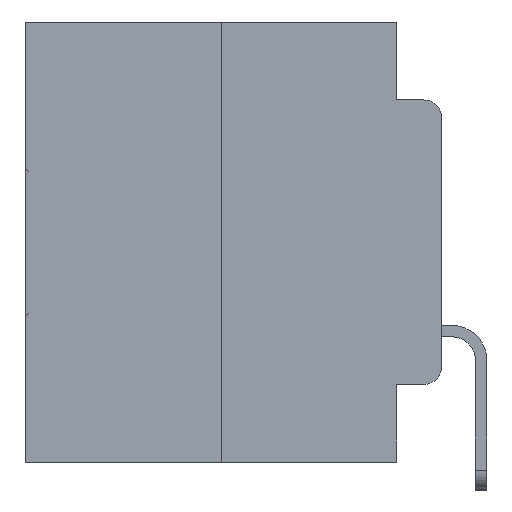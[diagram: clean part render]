
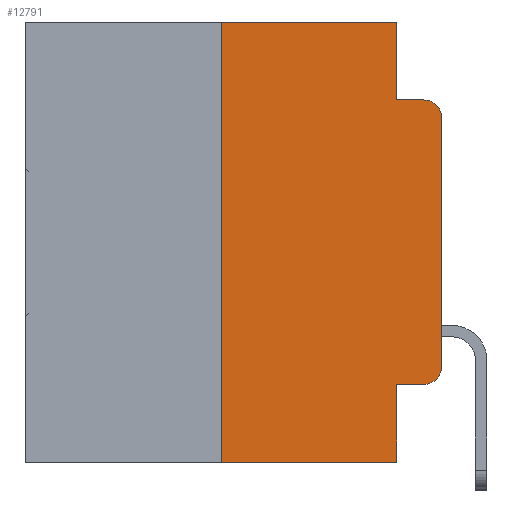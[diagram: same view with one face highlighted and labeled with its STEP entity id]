
A CAD part, left-side view. The second image highlights one B-rep face of the part: STEP entity #12791.
In plain terms, the highlighted planar face has unit normal (-1, 0, 0).
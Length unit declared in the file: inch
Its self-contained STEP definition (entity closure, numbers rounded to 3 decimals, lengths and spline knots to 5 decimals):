
#526 = DIRECTION ( 'NONE',  ( 0., -1., 0. ) ) ;
#586 = DIRECTION ( 'NONE',  ( 0., 0., -1. ) ) ;
#830 = CARTESIAN_POINT ( 'NONE',  ( 0., 0.02, -0.4115 ) ) ;
#928 = EDGE_CURVE ( 'NONE', #4862, #18999, #29889, .T. ) ;
#1311 = DIRECTION ( 'NONE',  ( -1., 0., 0. ) ) ;
#1475 = VECTOR ( 'NONE', #29833, 39.37008 ) ;
#1759 = CARTESIAN_POINT ( 'NONE',  ( 0., 0.473, -0.5 ) ) ;
#2125 = VERTEX_POINT ( 'NONE', #4407 ) ;
#2198 = FACE_OUTER_BOUND ( 'NONE', #23695, .T. ) ;
#2597 = LINE ( 'NONE', #1759, #7524 ) ;
#2882 = EDGE_CURVE ( 'NONE', #18999, #2125, #15155, .T. ) ;
#4063 = CARTESIAN_POINT ( 'NONE',  ( 0., 0.02, -0.0885 ) ) ;
#4392 = CARTESIAN_POINT ( 'NONE',  ( 0., 0., -0.3915 ) ) ;
#4407 = CARTESIAN_POINT ( 'NONE',  ( 0., 0., -0.1085 ) ) ;
#4862 = VERTEX_POINT ( 'NONE', #830 ) ;
#7303 = ORIENTED_EDGE ( 'NONE', *, *, #928, .T. ) ;
#7524 = VECTOR ( 'NONE', #16110, 39.37008 ) ;
#9722 = VECTOR ( 'NONE', #9874, 39.37008 ) ;
#9874 = DIRECTION ( 'NONE',  ( 0., 0., -1. ) ) ;
#9899 = DIRECTION ( 'NONE',  ( -1., 0., 0. ) ) ;
#10083 = VERTEX_POINT ( 'NONE', #19619 ) ;
#10897 = AXIS2_PLACEMENT_3D ( 'NONE', #15688, #1311, #18074 ) ;
#10962 = ORIENTED_EDGE ( 'NONE', *, *, #14187, .F. ) ;
#11020 = ORIENTED_EDGE ( 'NONE', *, *, #17382, .F. ) ;
#11183 = VECTOR ( 'NONE', #17807, 39.37008 ) ;
#11279 = CARTESIAN_POINT ( 'NONE',  ( 0., 0.473, 0. ) ) ;
#11471 = VECTOR ( 'NONE', #526, 39.37008 ) ;
#12084 = ORIENTED_EDGE ( 'NONE', *, *, #2882, .T. ) ;
#12791 = ADVANCED_FACE ( 'NONE', ( #2198 ), #28862, .F. ) ;
#12990 = EDGE_CURVE ( 'NONE', #2125, #17386, #26927, .T. ) ;
#13762 = CARTESIAN_POINT ( 'NONE',  ( 0., 0.051, -0.4115 ) ) ;
#13864 = DIRECTION ( 'NONE',  ( 0., -1., 0. ) ) ;
#13893 = CARTESIAN_POINT ( 'NONE',  ( 0., 0.051, -0.5 ) ) ;
#14046 = VECTOR ( 'NONE', #13864, 39.37008 ) ;
#14060 = ORIENTED_EDGE ( 'NONE', *, *, #23161, .F. ) ;
#14187 = EDGE_CURVE ( 'NONE', #14224, #10083, #23604, .T. ) ;
#14224 = VERTEX_POINT ( 'NONE', #15515 ) ;
#14301 = VERTEX_POINT ( 'NONE', #15720 ) ;
#14317 = CARTESIAN_POINT ( 'NONE',  ( 0., 0.051, 0. ) ) ;
#14913 = CARTESIAN_POINT ( 'NONE',  ( 0., 0.051, -0.0885 ) ) ;
#14995 = EDGE_CURVE ( 'NONE', #17907, #4862, #21019, .T. ) ;
#15155 = LINE ( 'NONE', #23709, #26784 ) ;
#15415 = CARTESIAN_POINT ( 'NONE',  ( 0., 0.25, 0. ) ) ;
#15423 = ORIENTED_EDGE ( 'NONE', *, *, #20666, .F. ) ;
#15515 = CARTESIAN_POINT ( 'NONE',  ( 0., 0.25, -0.5 ) ) ;
#15688 = CARTESIAN_POINT ( 'NONE',  ( 0., 0.02, -0.1085 ) ) ;
#15720 = CARTESIAN_POINT ( 'NONE',  ( 0., 0.051, -0.0885 ) ) ;
#16110 = DIRECTION ( 'NONE',  ( 0., -1., 0. ) ) ;
#16299 = VERTEX_POINT ( 'NONE', #13893 ) ;
#17382 = EDGE_CURVE ( 'NONE', #10083, #25867, #21231, .T. ) ;
#17386 = VERTEX_POINT ( 'NONE', #4063 ) ;
#17807 = DIRECTION ( 'NONE',  ( 0., 0., 1. ) ) ;
#17907 = VERTEX_POINT ( 'NONE', #18939 ) ;
#18074 = DIRECTION ( 'NONE',  ( 0., 0., -1. ) ) ;
#18330 = ORIENTED_EDGE ( 'NONE', *, *, #12990, .T. ) ;
#18939 = CARTESIAN_POINT ( 'NONE',  ( 0., 0.051, -0.4115 ) ) ;
#18999 = VERTEX_POINT ( 'NONE', #4392 ) ;
#19619 = CARTESIAN_POINT ( 'NONE',  ( 0., 0.25, 0. ) ) ;
#20666 = EDGE_CURVE ( 'NONE', #14301, #17386, #23881, .T. ) ;
#21019 = LINE ( 'NONE', #13762, #14046 ) ;
#21231 = LINE ( 'NONE', #11279, #1475 ) ;
#22764 = ORIENTED_EDGE ( 'NONE', *, *, #29150, .F. ) ;
#22912 = LINE ( 'NONE', #26207, #9722 ) ;
#23161 = EDGE_CURVE ( 'NONE', #25867, #14301, #30252, .T. ) ;
#23604 = LINE ( 'NONE', #15415, #11183 ) ;
#23695 = EDGE_LOOP ( 'NONE', ( #12084, #18330, #15423, #14060, #11020, #10962, #24296, #22764, #26747, #7303 ) ) ;
#23709 = CARTESIAN_POINT ( 'NONE',  ( 0., 0., 0. ) ) ;
#23881 = LINE ( 'NONE', #14913, #11471 ) ;
#23907 = CARTESIAN_POINT ( 'NONE',  ( 0., 0.02, -0.3915 ) ) ;
#24177 = VECTOR ( 'NONE', #28761, 39.37008 ) ;
#24296 = ORIENTED_EDGE ( 'NONE', *, *, #30319, .T. ) ;
#25867 = VERTEX_POINT ( 'NONE', #14317 ) ;
#26034 = DIRECTION ( 'NONE',  ( 0., 0., 1. ) ) ;
#26207 = CARTESIAN_POINT ( 'NONE',  ( 0., 0.051, 0. ) ) ;
#26242 = DIRECTION ( 'NONE',  ( 0., 0., -1. ) ) ;
#26472 = CARTESIAN_POINT ( 'NONE',  ( 0., 0.051, 0. ) ) ;
#26569 = CARTESIAN_POINT ( 'NONE',  ( 0., 0.473, 0. ) ) ;
#26747 = ORIENTED_EDGE ( 'NONE', *, *, #14995, .T. ) ;
#26784 = VECTOR ( 'NONE', #26034, 39.37008 ) ;
#26927 = CIRCLE ( 'NONE', #10897, 0.02 ) ;
#27095 = AXIS2_PLACEMENT_3D ( 'NONE', #26569, #28771, #586 ) ;
#28031 = AXIS2_PLACEMENT_3D ( 'NONE', #23907, #9899, #26242 ) ;
#28761 = DIRECTION ( 'NONE',  ( 0., 0., -1. ) ) ;
#28771 = DIRECTION ( 'NONE',  ( 1., 0., 0. ) ) ;
#28862 = PLANE ( 'NONE',  #27095 ) ;
#29150 = EDGE_CURVE ( 'NONE', #17907, #16299, #22912, .T. ) ;
#29833 = DIRECTION ( 'NONE',  ( 0., -1., 0. ) ) ;
#29889 = CIRCLE ( 'NONE', #28031, 0.02 ) ;
#30252 = LINE ( 'NONE', #26472, #24177 ) ;
#30319 = EDGE_CURVE ( 'NONE', #14224, #16299, #2597, .T. ) ;
